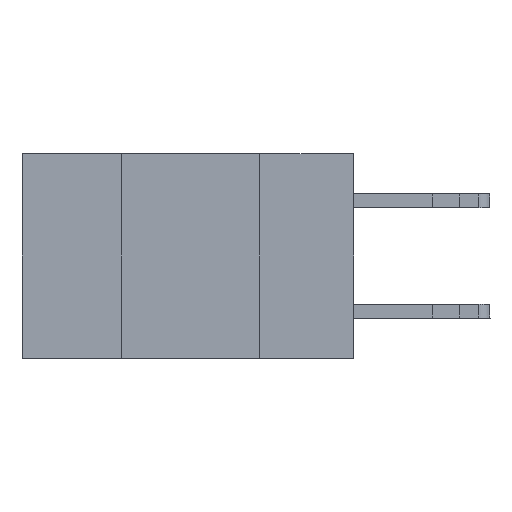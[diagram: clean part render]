
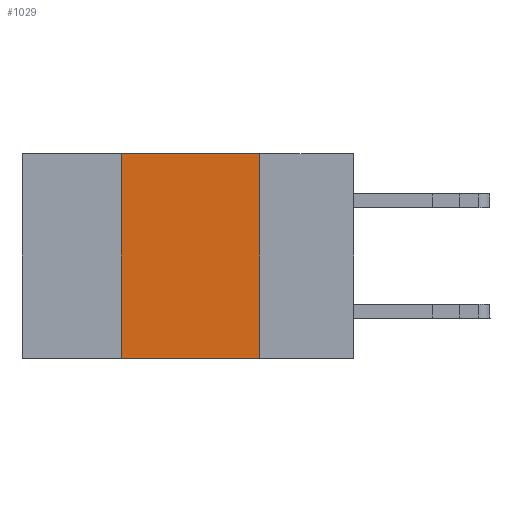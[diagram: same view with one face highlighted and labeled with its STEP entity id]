
A CAD part, left-side view. The second image highlights one B-rep face of the part: STEP entity #1029.
In plain terms, the highlighted planar face has unit normal (-1, 0, 0).
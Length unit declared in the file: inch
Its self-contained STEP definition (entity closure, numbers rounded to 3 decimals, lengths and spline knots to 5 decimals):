
#479 = CARTESIAN_POINT ( 'NONE',  ( 0., 0.6, -0.37 ) ) ;
#1029 = ADVANCED_FACE ( 'NONE', ( #17644 ), #1136, .F. ) ;
#1047 = DIRECTION ( 'NONE',  ( 0., 0., -1. ) ) ;
#1068 = DIRECTION ( 'NONE',  ( 1., 0., 0. ) ) ;
#1136 = PLANE ( 'NONE',  #11631 ) ;
#1310 = CARTESIAN_POINT ( 'NONE',  ( 0., 0.42, 0. ) ) ;
#1474 = CARTESIAN_POINT ( 'NONE',  ( 0., 0.6, 0. ) ) ;
#1865 = VECTOR ( 'NONE', #17282, 39.37008 ) ;
#1997 = CARTESIAN_POINT ( 'NONE',  ( 0., 0.17, -0.37 ) ) ;
#2290 = VECTOR ( 'NONE', #7851, 39.37008 ) ;
#2302 = ORIENTED_EDGE ( 'NONE', *, *, #2989, .F. ) ;
#2589 = LINE ( 'NONE', #479, #10558 ) ;
#2989 = EDGE_CURVE ( 'NONE', #10493, #15068, #6109, .T. ) ;
#3233 = ORIENTED_EDGE ( 'NONE', *, *, #11279, .F. ) ;
#3362 = CARTESIAN_POINT ( 'NONE',  ( 0., 0.17, 0. ) ) ;
#3574 = EDGE_LOOP ( 'NONE', ( #3233, #9621, #2302, #17696 ) ) ;
#6109 = LINE ( 'NONE', #1310, #1865 ) ;
#6366 = VECTOR ( 'NONE', #8527, 39.37008 ) ;
#7029 = EDGE_CURVE ( 'NONE', #15068, #15606, #19737, .T. ) ;
#7851 = DIRECTION ( 'NONE',  ( 0., -1., 0. ) ) ;
#7855 = VERTEX_POINT ( 'NONE', #1997 ) ;
#8527 = DIRECTION ( 'NONE',  ( 0., 0., -1. ) ) ;
#9621 = ORIENTED_EDGE ( 'NONE', *, *, #7029, .F. ) ;
#10070 = CARTESIAN_POINT ( 'NONE',  ( 0., 0.42, -0.37 ) ) ;
#10493 = VERTEX_POINT ( 'NONE', #10070 ) ;
#10558 = VECTOR ( 'NONE', #13345, 39.37008 ) ;
#10617 = LINE ( 'NONE', #16458, #6366 ) ;
#11279 = EDGE_CURVE ( 'NONE', #15606, #7855, #10617, .T. ) ;
#11631 = AXIS2_PLACEMENT_3D ( 'NONE', #1474, #1068, #1047 ) ;
#12599 = EDGE_CURVE ( 'NONE', #10493, #7855, #2589, .T. ) ;
#13345 = DIRECTION ( 'NONE',  ( 0., -1., 0. ) ) ;
#14368 = CARTESIAN_POINT ( 'NONE',  ( 0., 0.42, 0. ) ) ;
#15068 = VERTEX_POINT ( 'NONE', #14368 ) ;
#15606 = VERTEX_POINT ( 'NONE', #3362 ) ;
#15889 = CARTESIAN_POINT ( 'NONE',  ( 0., 0.6, 0. ) ) ;
#16458 = CARTESIAN_POINT ( 'NONE',  ( 0., 0.17, 0. ) ) ;
#17282 = DIRECTION ( 'NONE',  ( 0., 0., 1. ) ) ;
#17644 = FACE_OUTER_BOUND ( 'NONE', #3574, .T. ) ;
#17696 = ORIENTED_EDGE ( 'NONE', *, *, #12599, .T. ) ;
#19737 = LINE ( 'NONE', #15889, #2290 ) ;
